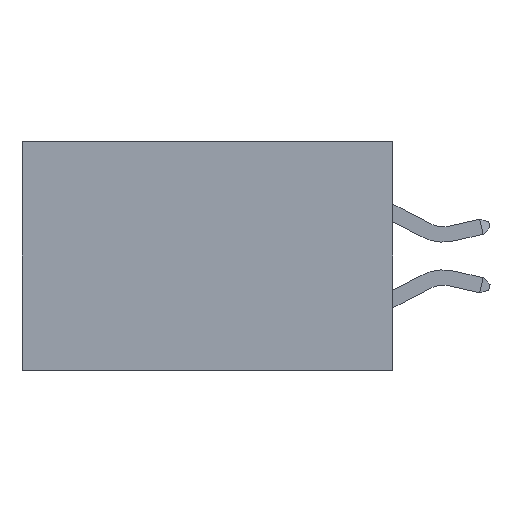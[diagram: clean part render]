
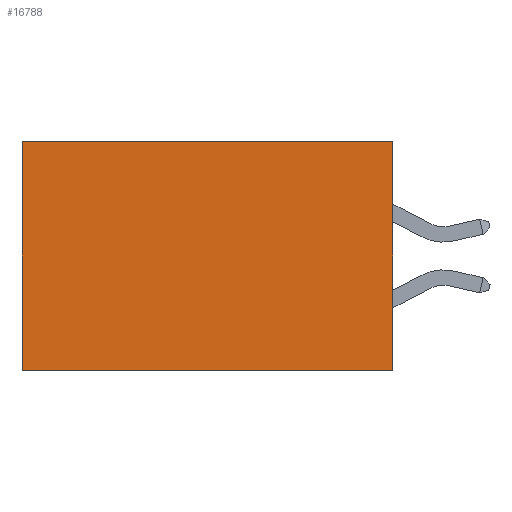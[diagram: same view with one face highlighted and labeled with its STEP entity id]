
A CAD part, left-side view. The second image highlights one B-rep face of the part: STEP entity #16788.
In plain terms, the highlighted planar face has unit normal (-1, 0, 0).
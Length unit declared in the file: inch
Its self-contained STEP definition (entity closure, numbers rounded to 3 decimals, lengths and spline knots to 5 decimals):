
#1040 = LINE ( 'NONE', #5057, #29284 ) ;
#1902 = CARTESIAN_POINT ( 'NONE',  ( 0.2875, 0., 0. ) ) ;
#1976 = VERTEX_POINT ( 'NONE', #17945 ) ;
#2128 = EDGE_CURVE ( 'NONE', #26461, #15018, #7293, .T. ) ;
#2757 = DIRECTION ( 'NONE',  ( 0., 0., -1. ) ) ;
#3345 = AXIS2_PLACEMENT_3D ( 'NONE', #27078, #21431, #24472 ) ;
#3349 = LINE ( 'NONE', #1902, #10950 ) ;
#5057 = CARTESIAN_POINT ( 'NONE',  ( 0.2875, 0.6, 0. ) ) ;
#7293 = LINE ( 'NONE', #32206, #24623 ) ;
#7506 = EDGE_CURVE ( 'NONE', #1976, #21577, #1040, .T. ) ;
#7886 = DIRECTION ( 'NONE',  ( 0., 0., -1. ) ) ;
#8700 = CARTESIAN_POINT ( 'NONE',  ( 0.2875, 0., 0. ) ) ;
#9126 = VECTOR ( 'NONE', #18419, 39.37008 ) ;
#10950 = VECTOR ( 'NONE', #18125, 39.37008 ) ;
#11016 = PLANE ( 'NONE',  #3345 ) ;
#11883 = CARTESIAN_POINT ( 'NONE',  ( 0.2875, 0., -0.37 ) ) ;
#12955 = ORIENTED_EDGE ( 'NONE', *, *, #7506, .T. ) ;
#15018 = VERTEX_POINT ( 'NONE', #22082 ) ;
#15193 = EDGE_LOOP ( 'NONE', ( #12955, #20707, #26737, #21904 ) ) ;
#16788 = ADVANCED_FACE ( 'NONE', ( #23269 ), #11016, .F. ) ;
#17368 = CARTESIAN_POINT ( 'NONE',  ( 0.2875, 0.6, -0.37 ) ) ;
#17945 = CARTESIAN_POINT ( 'NONE',  ( 0.2875, 0.6, 0. ) ) ;
#18125 = DIRECTION ( 'NONE',  ( 0., 1., 0. ) ) ;
#18419 = DIRECTION ( 'NONE',  ( 0., 1., 0. ) ) ;
#19831 = EDGE_CURVE ( 'NONE', #15018, #21577, #25628, .T. ) ;
#20707 = ORIENTED_EDGE ( 'NONE', *, *, #19831, .F. ) ;
#21431 = DIRECTION ( 'NONE',  ( 1., 0., 0. ) ) ;
#21577 = VERTEX_POINT ( 'NONE', #17368 ) ;
#21904 = ORIENTED_EDGE ( 'NONE', *, *, #30190, .T. ) ;
#22082 = CARTESIAN_POINT ( 'NONE',  ( 0.2875, 0., -0.37 ) ) ;
#23269 = FACE_OUTER_BOUND ( 'NONE', #15193, .T. ) ;
#24472 = DIRECTION ( 'NONE',  ( 0., 0., -1. ) ) ;
#24623 = VECTOR ( 'NONE', #2757, 39.37008 ) ;
#25628 = LINE ( 'NONE', #11883, #9126 ) ;
#26461 = VERTEX_POINT ( 'NONE', #8700 ) ;
#26737 = ORIENTED_EDGE ( 'NONE', *, *, #2128, .F. ) ;
#27078 = CARTESIAN_POINT ( 'NONE',  ( 0.2875, 0., 0. ) ) ;
#29284 = VECTOR ( 'NONE', #7886, 39.37008 ) ;
#30190 = EDGE_CURVE ( 'NONE', #26461, #1976, #3349, .T. ) ;
#32206 = CARTESIAN_POINT ( 'NONE',  ( 0.2875, 0., 0. ) ) ;
